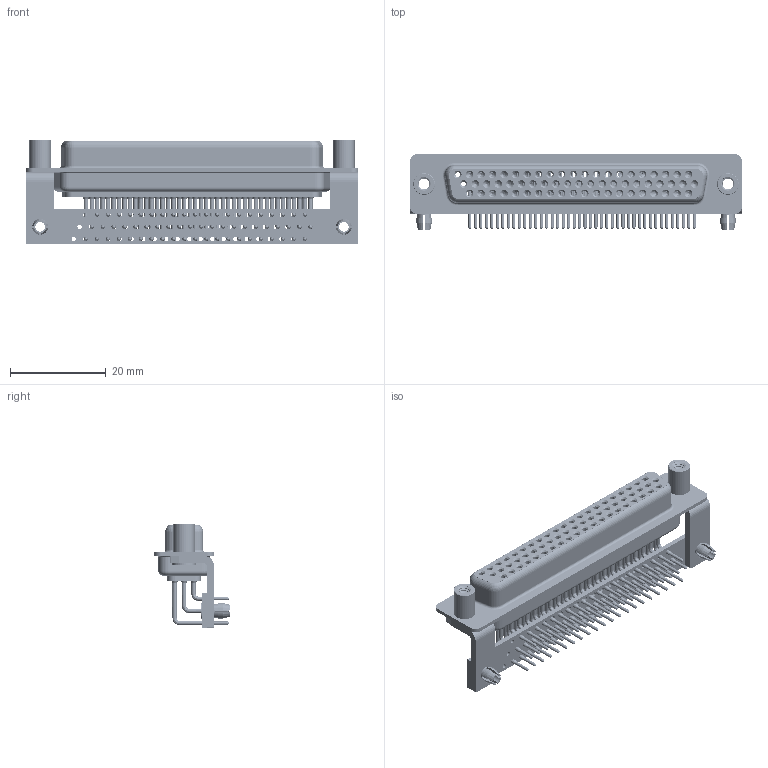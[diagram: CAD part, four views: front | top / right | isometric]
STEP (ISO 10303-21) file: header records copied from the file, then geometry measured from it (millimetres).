
FILE_DESCRIPTION (( 'STEP AP203' ), '1' );
FILE_NAME ('634-M62-663-BN5.STEP', '2018-09-28T03:59:18', ( '' ), ( '' ), 'SwSTEP 2.0', 'SolidWorks 2016', '' );
FILE_SCHEMA (( 'CONFIG_CONTROL_DESIGN' ));
Length unit declared in the file: millimetre
Products named in the file (11): 634M Housing_62 Contacts; 634M Stabilizer Board_62 Contacts; 634M Shell Front_62 Contacts; 634M Board Lock; 634M Shell Rear_62 Contacts; 634-M62-663-BN5; 634M Contact Row 1; 634M Contact Row 2; 634M Contact Row 3; 634M Stabilizer Bracket; 634M 4-40 Threaded Standoff
Assembly tree (72 placements, depth 2):
  634-M62-663-BN5
    634M Housing_62 Contacts
    634M Shell Front_62 Contacts
    634M Shell Rear_62 Contacts
    634M Contact Row 1  x21
    634M Contact Row 2  x21
    634M Contact Row 3  x20
    634M Stabilizer Bracket  x2
    634M 4-40 Threaded Standoff  x2
    634M Stabilizer Board_62 Contacts
    634M Board Lock  x2
Bounding box: 69.4 x 15.8 x 21.9 mm (x, y, z)
Volume: 6304.5 mm3; surface area: 20283.8 mm2
Topology: 72 solids, 72 shells, 3881 faces, 9941 edges, 6283 vertices
Faces by surface type: cylinder 1783, plane 1073, cone 708, bspline 254, torus 63
Entity records: 46472 total; most frequent: CARTESIAN_POINT 9257, DIRECTION 7957, ORIENTED_EDGE 6580, AXIS2_PLACEMENT_3D 3353, EDGE_CURVE 3290, VERTEX_POINT 2117, CIRCLE 1896, EDGE_LOOP 1873
